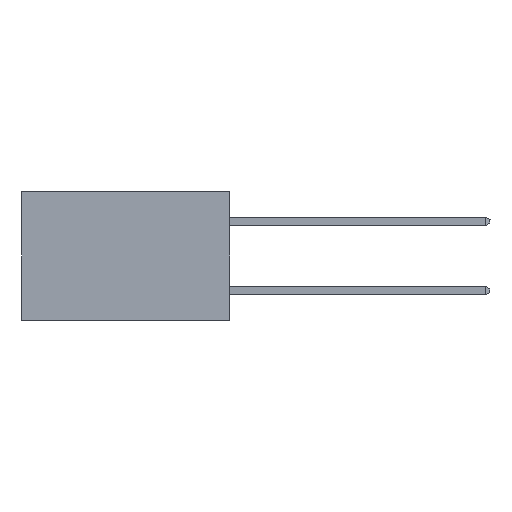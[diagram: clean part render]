
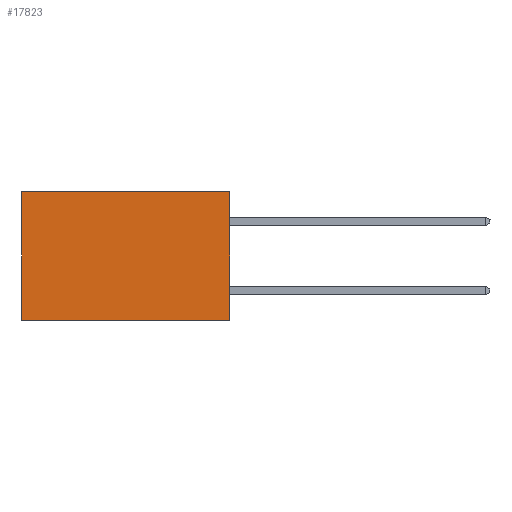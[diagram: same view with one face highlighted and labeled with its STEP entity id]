
A CAD part, left-side view. The second image highlights one B-rep face of the part: STEP entity #17823.
In plain terms, the highlighted planar face has unit normal (-1, 0, 0).
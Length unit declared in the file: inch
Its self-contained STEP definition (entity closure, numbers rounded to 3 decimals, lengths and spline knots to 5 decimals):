
#1569 = DIRECTION ( 'NONE',  ( 0., 0., -1. ) ) ;
#2586 = CARTESIAN_POINT ( 'NONE',  ( 0.298, 0.6, -0.37 ) ) ;
#3383 = EDGE_CURVE ( 'NONE', #6763, #9556, #21154, .T. ) ;
#4376 = ORIENTED_EDGE ( 'NONE', *, *, #6419, .T. ) ;
#5311 = VECTOR ( 'NONE', #23611, 39.37008 ) ;
#6148 = CARTESIAN_POINT ( 'NONE',  ( 0.298, 0., -0.37 ) ) ;
#6419 = EDGE_CURVE ( 'NONE', #11391, #17657, #23316, .T. ) ;
#6634 = DIRECTION ( 'NONE',  ( 0., 1., 0. ) ) ;
#6763 = VERTEX_POINT ( 'NONE', #25223 ) ;
#6839 = VECTOR ( 'NONE', #28059, 39.37008 ) ;
#6973 = LINE ( 'NONE', #16035, #5311 ) ;
#9556 = VERTEX_POINT ( 'NONE', #2586 ) ;
#10356 = EDGE_CURVE ( 'NONE', #11391, #6763, #23546, .T. ) ;
#11391 = VERTEX_POINT ( 'NONE', #12020 ) ;
#12020 = CARTESIAN_POINT ( 'NONE',  ( 0.298, 0., 0. ) ) ;
#13070 = CARTESIAN_POINT ( 'NONE',  ( 0.298, 0., 0. ) ) ;
#13175 = DIRECTION ( 'NONE',  ( 0., 0., -1. ) ) ;
#16035 = CARTESIAN_POINT ( 'NONE',  ( 0.298, 0.6, 0. ) ) ;
#16993 = DIRECTION ( 'NONE',  ( 1., 0., 0. ) ) ;
#17657 = VERTEX_POINT ( 'NONE', #21266 ) ;
#17823 = ADVANCED_FACE ( 'NONE', ( #26752 ), #29557, .F. ) ;
#19100 = EDGE_LOOP ( 'NONE', ( #24518, #23265, #23137, #4376 ) ) ;
#21154 = LINE ( 'NONE', #6148, #6839 ) ;
#21266 = CARTESIAN_POINT ( 'NONE',  ( 0.298, 0.6, 0. ) ) ;
#21980 = AXIS2_PLACEMENT_3D ( 'NONE', #32052, #16993, #1569 ) ;
#22769 = VECTOR ( 'NONE', #13175, 39.37008 ) ;
#23137 = ORIENTED_EDGE ( 'NONE', *, *, #10356, .F. ) ;
#23265 = ORIENTED_EDGE ( 'NONE', *, *, #3383, .F. ) ;
#23316 = LINE ( 'NONE', #24418, #30050 ) ;
#23546 = LINE ( 'NONE', #13070, #22769 ) ;
#23611 = DIRECTION ( 'NONE',  ( 0., 0., -1. ) ) ;
#24044 = EDGE_CURVE ( 'NONE', #17657, #9556, #6973, .T. ) ;
#24418 = CARTESIAN_POINT ( 'NONE',  ( 0.298, 0., 0. ) ) ;
#24518 = ORIENTED_EDGE ( 'NONE', *, *, #24044, .T. ) ;
#25223 = CARTESIAN_POINT ( 'NONE',  ( 0.298, 0., -0.37 ) ) ;
#26752 = FACE_OUTER_BOUND ( 'NONE', #19100, .T. ) ;
#28059 = DIRECTION ( 'NONE',  ( 0., 1., 0. ) ) ;
#29557 = PLANE ( 'NONE',  #21980 ) ;
#30050 = VECTOR ( 'NONE', #6634, 39.37008 ) ;
#32052 = CARTESIAN_POINT ( 'NONE',  ( 0.298, 0., 0. ) ) ;
